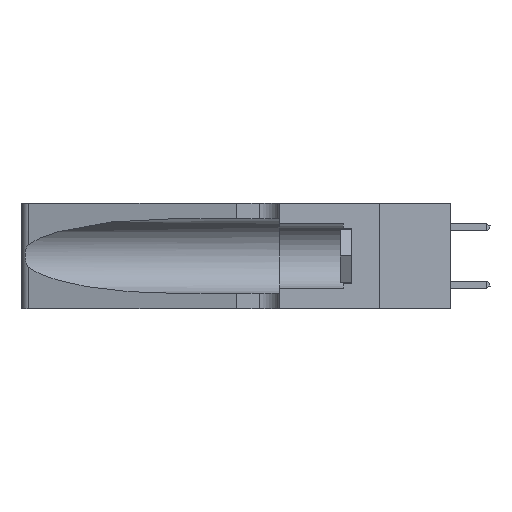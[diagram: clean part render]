
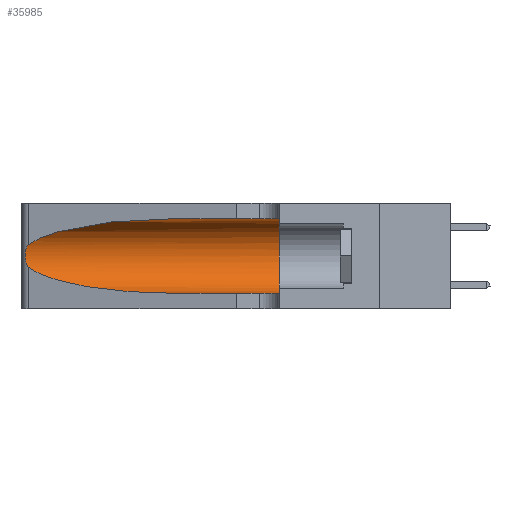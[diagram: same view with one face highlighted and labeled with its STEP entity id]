
A CAD part, left-side view. The second image highlights one B-rep face of the part: STEP entity #35985.
In plain terms, the highlighted cylindrical face has radius 3.308 mm (diameter 6.617 mm), a partial arc.
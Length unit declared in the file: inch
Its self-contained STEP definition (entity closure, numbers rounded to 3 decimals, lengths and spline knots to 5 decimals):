
#1937 = ORIENTED_EDGE ( 'NONE', *, *, #16225, .T. ) ;
#2183 = CARTESIAN_POINT ( 'NONE',  ( 0.26018, 1.23835, 0.19895 ) ) ;
#2379 =( BOUNDED_CURVE ( )  B_SPLINE_CURVE ( 3, ( #24382, #36887, #30680, #11804 ),
 .UNSPECIFIED., .F., .F. ) 
 B_SPLINE_CURVE_WITH_KNOTS ( ( 4, 4 ),
 ( 1.5708, 2.84003 ),
 .UNSPECIFIED. ) 
 CURVE ( )  GEOMETRIC_REPRESENTATION_ITEM ( )  RATIONAL_B_SPLINE_CURVE ( ( 1., 0.87, 0.87, 1. ) ) 
 REPRESENTATION_ITEM ( '' )  );
#2763 = EDGE_CURVE ( 'NONE', #36601, #14504, #25813, .T. ) ;
#3359 = ORIENTED_EDGE ( 'NONE', *, *, #4873, .T. ) ;
#4873 = EDGE_CURVE ( 'NONE', #10731, #14504, #16778, .T. ) ;
#5417 = CARTESIAN_POINT ( 'NONE',  ( 0.26075, 1.23896, 0.178 ) ) ;
#5427 = CARTESIAN_POINT ( 'NONE',  ( 0.25487, 1.22718, 0.22369 ) ) ;
#5663 = ORIENTED_EDGE ( 'NONE', *, *, #19797, .T. ) ;
#5965 = EDGE_CURVE ( 'NONE', #25348, #10731, #31830, .T. ) ;
#5966 = CARTESIAN_POINT ( 'NONE',  ( 0.1305, 0.72297, 0.05475 ) ) ;
#6108 = CARTESIAN_POINT ( 'NONE',  ( 0.1305, 0.35, 0.185 ) ) ;
#8315 = CARTESIAN_POINT ( 'NONE',  ( 0.18966, 0.96281, 0.05475 ) ) ;
#8601 = CARTESIAN_POINT ( 'NONE',  ( 0.25856, 1.23593, 0.16098 ) ) ;
#9305 = DIRECTION ( 'NONE',  ( 0., 0., 1. ) ) ;
#10731 = VERTEX_POINT ( 'NONE', #5966 ) ;
#11804 = CARTESIAN_POINT ( 'NONE',  ( 0.25487, 1.22718, 0.22369 ) ) ;
#11835 = CARTESIAN_POINT ( 'NONE',  ( 0.25639, 1.23186, 0.15144 ) ) ;
#12200 = CARTESIAN_POINT ( 'NONE',  ( 0.1305, 0.35, 0.05475 ) ) ;
#12268 = CYLINDRICAL_SURFACE ( 'NONE', #15180, 0.13025 ) ;
#12376 = DIRECTION ( 'NONE',  ( 0., -1., 0. ) ) ;
#12785 = DIRECTION ( 'NONE',  ( 0., -1., 0. ) ) ;
#13955 = VERTEX_POINT ( 'NONE', #5427 ) ;
#14192 = EDGE_CURVE ( 'NONE', #24360, #36601, #26225, .T. ) ;
#14504 = VERTEX_POINT ( 'NONE', #12200 ) ;
#14711 = CARTESIAN_POINT ( 'NONE',  ( 0.25487, 1.22718, 0.14631 ) ) ;
#14865 = CARTESIAN_POINT ( 'NONE',  ( 0.25487, 1.22718, 0.22369 ) ) ;
#15004 = CARTESIAN_POINT ( 'NONE',  ( 0.25487, 1.22718, 0.14631 ) ) ;
#15180 = AXIS2_PLACEMENT_3D ( 'NONE', #22267, #31722, #38061 ) ;
#16225 = EDGE_CURVE ( 'NONE', #24360, #13955, #2379, .T. ) ;
#16578 = ORIENTED_EDGE ( 'NONE', *, *, #2763, .F. ) ;
#16621 = ORIENTED_EDGE ( 'NONE', *, *, #14192, .F. ) ;
#16778 = LINE ( 'NONE', #31244, #40877 ) ;
#16845 = EDGE_LOOP ( 'NONE', ( #1937, #5663, #35390, #3359, #16578, #16621 ) ) ;
#18067 = CARTESIAN_POINT ( 'NONE',  ( 0.25639, 1.23184, 0.21858 ) ) ;
#18294 = CARTESIAN_POINT ( 'NONE',  ( 0.1305, 0.72297, 0.31525 ) ) ;
#18852 = VECTOR ( 'NONE', #12785, 39.37008 ) ;
#19797 = EDGE_CURVE ( 'NONE', #13955, #25348, #28800, .T. ) ;
#21250 = CARTESIAN_POINT ( 'NONE',  ( 0.25854, 1.2359, 0.20912 ) ) ;
#22267 = CARTESIAN_POINT ( 'NONE',  ( 0.1305, 1.61858, 0.185 ) ) ;
#24360 = VERTEX_POINT ( 'NONE', #18294 ) ;
#24382 = CARTESIAN_POINT ( 'NONE',  ( 0.1305, 0.72297, 0.31525 ) ) ;
#24417 = CARTESIAN_POINT ( 'NONE',  ( 0.26075, 1.23896, 0.19203 ) ) ;
#25348 = VERTEX_POINT ( 'NONE', #26199 ) ;
#25813 = CIRCLE ( 'NONE', #34923, 0.13025 ) ;
#26199 = CARTESIAN_POINT ( 'NONE',  ( 0.25487, 1.22718, 0.14631 ) ) ;
#26225 = LINE ( 'NONE', #28509, #18852 ) ;
#27543 = CARTESIAN_POINT ( 'NONE',  ( 0.26017, 1.23833, 0.17102 ) ) ;
#28245 = DIRECTION ( 'NONE',  ( 0., 1., 0. ) ) ;
#28509 = CARTESIAN_POINT ( 'NONE',  ( 0.1305, 1.61858, 0.31525 ) ) ;
#28800 = B_SPLINE_CURVE_WITH_KNOTS ( 'NONE', 3,
 ( #14865, #33717, #18067, #40070, #21250, #2183, #24417, #5417, #27543, #8601, #30711, #11835, #33855, #15004 ),
 .UNSPECIFIED., .F., .F.,
 ( 4, 2, 2, 2, 2, 2, 4 ),
 ( 0., 0.00027, 0.00053, 0.00107, 0.0016, 0.00187, 0.00214 ),
 .UNSPECIFIED. ) ;
#29031 = FACE_OUTER_BOUND ( 'NONE', #16845, .T. ) ;
#30680 = CARTESIAN_POINT ( 'NONE',  ( 0.2373, 1.15595, 0.28018 ) ) ;
#30711 = CARTESIAN_POINT ( 'NONE',  ( 0.25789, 1.23486, 0.15765 ) ) ;
#31244 = CARTESIAN_POINT ( 'NONE',  ( 0.1305, 1.61858, 0.05475 ) ) ;
#31384 = CARTESIAN_POINT ( 'NONE',  ( 0.1305, 0.35, 0.31525 ) ) ;
#31722 = DIRECTION ( 'NONE',  ( 0., -1., 0. ) ) ;
#31830 =( BOUNDED_CURVE ( )  B_SPLINE_CURVE ( 3, ( #14711, #33573, #8315, #36773 ),
 .UNSPECIFIED., .F., .F. ) 
 B_SPLINE_CURVE_WITH_KNOTS ( ( 4, 4 ),
 ( 3.44316, 4.71239 ),
 .UNSPECIFIED. ) 
 CURVE ( )  GEOMETRIC_REPRESENTATION_ITEM ( )  RATIONAL_B_SPLINE_CURVE ( ( 1., 0.87, 0.87, 1. ) ) 
 REPRESENTATION_ITEM ( '' )  );
#33573 = CARTESIAN_POINT ( 'NONE',  ( 0.2373, 1.15595, 0.08982 ) ) ;
#33717 = CARTESIAN_POINT ( 'NONE',  ( 0.25555, 1.22994, 0.2215 ) ) ;
#33855 = CARTESIAN_POINT ( 'NONE',  ( 0.25555, 1.22993, 0.14849 ) ) ;
#34923 = AXIS2_PLACEMENT_3D ( 'NONE', #6108, #28245, #9305 ) ;
#35390 = ORIENTED_EDGE ( 'NONE', *, *, #5965, .T. ) ;
#35985 = ADVANCED_FACE ( 'NONE', ( #29031 ), #12268, .F. ) ;
#36601 = VERTEX_POINT ( 'NONE', #31384 ) ;
#36773 = CARTESIAN_POINT ( 'NONE',  ( 0.1305, 0.72297, 0.05475 ) ) ;
#36887 = CARTESIAN_POINT ( 'NONE',  ( 0.18966, 0.96281, 0.31525 ) ) ;
#38061 = DIRECTION ( 'NONE',  ( 0., 0., -1. ) ) ;
#40070 = CARTESIAN_POINT ( 'NONE',  ( 0.25787, 1.23484, 0.2124 ) ) ;
#40877 = VECTOR ( 'NONE', #12376, 39.37008 ) ;
